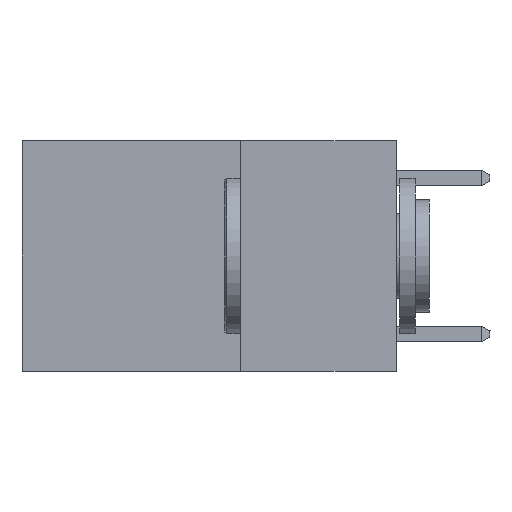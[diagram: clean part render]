
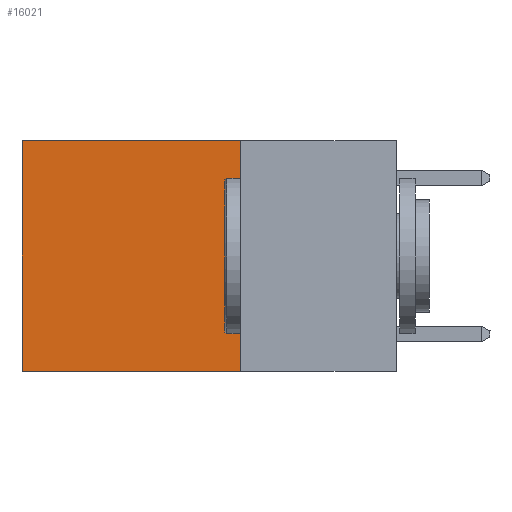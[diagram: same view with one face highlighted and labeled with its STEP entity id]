
A CAD part, left-side view. The second image highlights one B-rep face of the part: STEP entity #16021.
In plain terms, the highlighted planar face has unit normal (-1, 0, 0).
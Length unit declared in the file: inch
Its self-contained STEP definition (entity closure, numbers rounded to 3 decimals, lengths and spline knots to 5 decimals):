
#327 = EDGE_CURVE ( 'NONE', #12097, #5317, #13955, .T. ) ;
#1152 = AXIS2_PLACEMENT_3D ( 'NONE', #8194, #30714, #7869 ) ;
#1215 = CARTESIAN_POINT ( 'NONE',  ( 0.2625, 0.25, -0.37 ) ) ;
#1331 = DIRECTION ( 'NONE',  ( 0., 0., -1. ) ) ;
#1524 = LINE ( 'NONE', #9118, #4443 ) ;
#2904 = VECTOR ( 'NONE', #1331, 39.37008 ) ;
#3645 = LINE ( 'NONE', #20870, #2904 ) ;
#4443 = VECTOR ( 'NONE', #24692, 39.37008 ) ;
#5317 = VERTEX_POINT ( 'NONE', #14480 ) ;
#5849 = EDGE_CURVE ( 'NONE', #13074, #12097, #1524, .T. ) ;
#6127 = EDGE_CURVE ( 'NONE', #30903, #5317, #3645, .T. ) ;
#7085 = ORIENTED_EDGE ( 'NONE', *, *, #327, .F. ) ;
#7869 = DIRECTION ( 'NONE',  ( 0., 0., -1. ) ) ;
#8003 = EDGE_LOOP ( 'NONE', ( #18920, #7085, #18474, #10365 ) ) ;
#8194 = CARTESIAN_POINT ( 'NONE',  ( 0.2625, 0.25, 0. ) ) ;
#9118 = CARTESIAN_POINT ( 'NONE',  ( 0.2625, 0.25, 0. ) ) ;
#9736 = VECTOR ( 'NONE', #15981, 39.37008 ) ;
#10365 = ORIENTED_EDGE ( 'NONE', *, *, #20137, .T. ) ;
#12097 = VERTEX_POINT ( 'NONE', #27304 ) ;
#12843 = PLANE ( 'NONE',  #1152 ) ;
#13004 = FACE_OUTER_BOUND ( 'NONE', #8003, .T. ) ;
#13074 = VERTEX_POINT ( 'NONE', #15409 ) ;
#13955 = LINE ( 'NONE', #1215, #32398 ) ;
#14480 = CARTESIAN_POINT ( 'NONE',  ( 0.2625, 0.6, -0.37 ) ) ;
#15409 = CARTESIAN_POINT ( 'NONE',  ( 0.2625, 0.25, 0. ) ) ;
#15489 = CARTESIAN_POINT ( 'NONE',  ( 0.2625, 0.25, 0. ) ) ;
#15981 = DIRECTION ( 'NONE',  ( 0., 1., 0. ) ) ;
#16021 = ADVANCED_FACE ( 'NONE', ( #13004 ), #12843, .F. ) ;
#18474 = ORIENTED_EDGE ( 'NONE', *, *, #5849, .F. ) ;
#18657 = CARTESIAN_POINT ( 'NONE',  ( 0.2625, 0.6, 0. ) ) ;
#18920 = ORIENTED_EDGE ( 'NONE', *, *, #6127, .T. ) ;
#20137 = EDGE_CURVE ( 'NONE', #13074, #30903, #25587, .T. ) ;
#20870 = CARTESIAN_POINT ( 'NONE',  ( 0.2625, 0.6, 0. ) ) ;
#21562 = DIRECTION ( 'NONE',  ( 0., 1., 0. ) ) ;
#24692 = DIRECTION ( 'NONE',  ( 0., 0., -1. ) ) ;
#25587 = LINE ( 'NONE', #15489, #9736 ) ;
#27304 = CARTESIAN_POINT ( 'NONE',  ( 0.2625, 0.25, -0.37 ) ) ;
#30714 = DIRECTION ( 'NONE',  ( 1., 0., 0. ) ) ;
#30903 = VERTEX_POINT ( 'NONE', #18657 ) ;
#32398 = VECTOR ( 'NONE', #21562, 39.37008 ) ;
